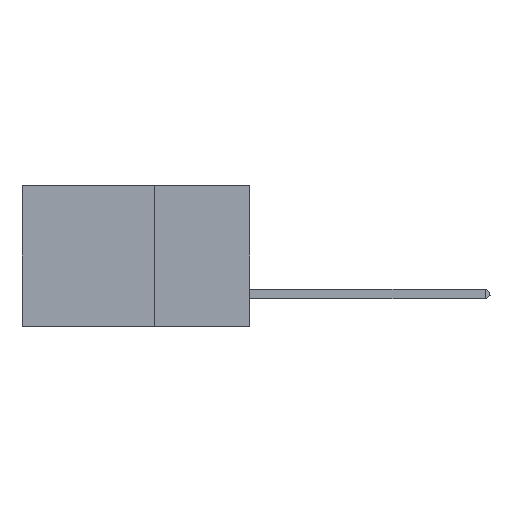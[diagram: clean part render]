
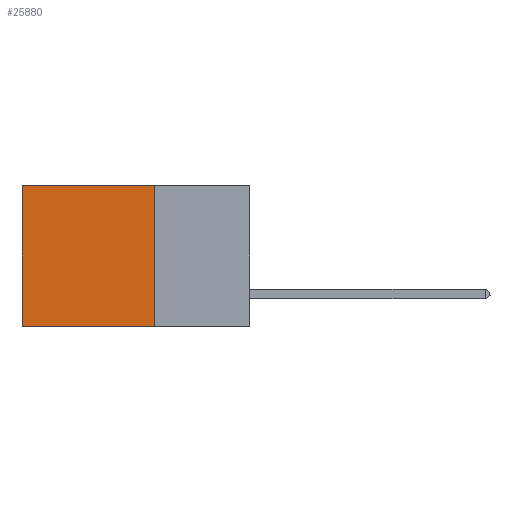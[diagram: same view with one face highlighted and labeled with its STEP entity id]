
A CAD part, left-side view. The second image highlights one B-rep face of the part: STEP entity #25880.
In plain terms, the highlighted planar face has unit normal (-1, 0, 0).
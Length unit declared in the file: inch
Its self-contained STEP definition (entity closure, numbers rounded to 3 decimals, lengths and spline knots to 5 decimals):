
#94 = EDGE_CURVE ( 'NONE', #24703, #20049, #13691, .T. ) ;
#831 = CARTESIAN_POINT ( 'NONE',  ( 0.2875, 0.25, 0. ) ) ;
#1210 = DIRECTION ( 'NONE',  ( 0., 0., -1. ) ) ;
#2085 = EDGE_LOOP ( 'NONE', ( #19370, #33864, #11944, #21535 ) ) ;
#2948 = EDGE_CURVE ( 'NONE', #20049, #26553, #31925, .T. ) ;
#5024 = EDGE_CURVE ( 'NONE', #23859, #26553, #9538, .T. ) ;
#5436 = CARTESIAN_POINT ( 'NONE',  ( 0.2875, 0.25, -0.37 ) ) ;
#5861 = CARTESIAN_POINT ( 'NONE',  ( 0.2875, 0.25, 0. ) ) ;
#9465 = DIRECTION ( 'NONE',  ( 1., 0., 0. ) ) ;
#9538 = LINE ( 'NONE', #15599, #14546 ) ;
#11801 = DIRECTION ( 'NONE',  ( 0., 0., -1. ) ) ;
#11944 = ORIENTED_EDGE ( 'NONE', *, *, #22219, .F. ) ;
#12867 = CARTESIAN_POINT ( 'NONE',  ( 0.2875, 0.6, 0. ) ) ;
#13440 = DIRECTION ( 'NONE',  ( 0., 0., -1. ) ) ;
#13691 = LINE ( 'NONE', #32469, #27079 ) ;
#14415 = CARTESIAN_POINT ( 'NONE',  ( 0.2875, 0.6, 0. ) ) ;
#14546 = VECTOR ( 'NONE', #26326, 39.37008 ) ;
#15397 = FACE_OUTER_BOUND ( 'NONE', #2085, .T. ) ;
#15599 = CARTESIAN_POINT ( 'NONE',  ( 0.2875, 0.25, -0.37 ) ) ;
#17671 = VECTOR ( 'NONE', #1210, 39.37008 ) ;
#18988 = VECTOR ( 'NONE', #13440, 39.37008 ) ;
#19370 = ORIENTED_EDGE ( 'NONE', *, *, #2948, .T. ) ;
#19741 = CARTESIAN_POINT ( 'NONE',  ( 0.2875, 0.25, 0. ) ) ;
#20049 = VERTEX_POINT ( 'NONE', #12867 ) ;
#21535 = ORIENTED_EDGE ( 'NONE', *, *, #94, .T. ) ;
#22219 = EDGE_CURVE ( 'NONE', #24703, #23859, #22769, .T. ) ;
#22558 = PLANE ( 'NONE',  #31587 ) ;
#22636 = CARTESIAN_POINT ( 'NONE',  ( 0.2875, 0.6, -0.37 ) ) ;
#22769 = LINE ( 'NONE', #5861, #18988 ) ;
#23859 = VERTEX_POINT ( 'NONE', #5436 ) ;
#24663 = DIRECTION ( 'NONE',  ( 0., 1., 0. ) ) ;
#24703 = VERTEX_POINT ( 'NONE', #831 ) ;
#25880 = ADVANCED_FACE ( 'NONE', ( #15397 ), #22558, .F. ) ;
#26326 = DIRECTION ( 'NONE',  ( 0., 1., 0. ) ) ;
#26553 = VERTEX_POINT ( 'NONE', #22636 ) ;
#27079 = VECTOR ( 'NONE', #24663, 39.37008 ) ;
#31587 = AXIS2_PLACEMENT_3D ( 'NONE', #19741, #9465, #11801 ) ;
#31925 = LINE ( 'NONE', #14415, #17671 ) ;
#32469 = CARTESIAN_POINT ( 'NONE',  ( 0.2875, 0.25, 0. ) ) ;
#33864 = ORIENTED_EDGE ( 'NONE', *, *, #5024, .F. ) ;
